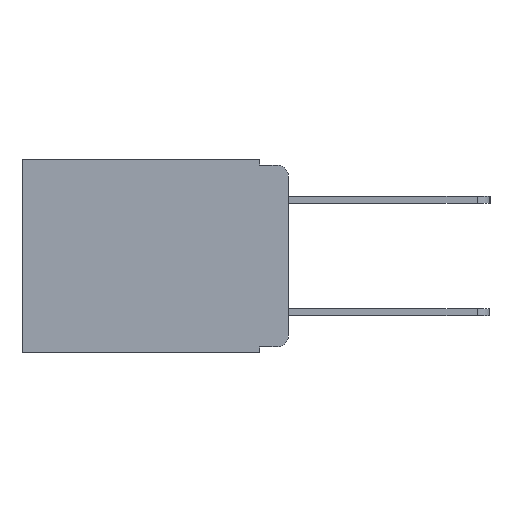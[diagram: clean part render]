
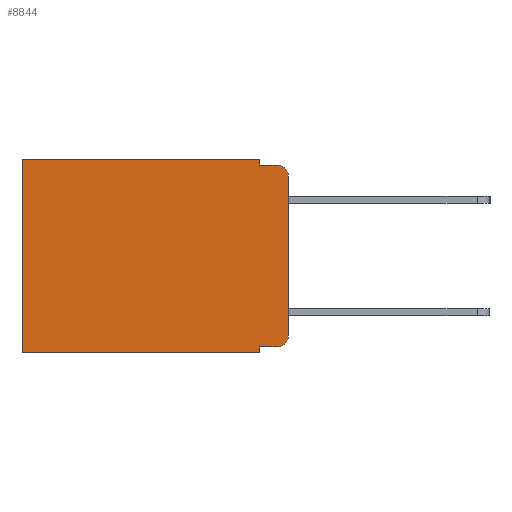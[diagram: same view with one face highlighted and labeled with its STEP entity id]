
A CAD part, left-side view. The second image highlights one B-rep face of the part: STEP entity #8844.
In plain terms, the highlighted planar face has unit normal (-1, 0, 0).
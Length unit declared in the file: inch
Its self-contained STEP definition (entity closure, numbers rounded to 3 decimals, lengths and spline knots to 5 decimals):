
#23 = FACE_OUTER_BOUND ( 'NONE', #2039, .T. ) ;
#120 = CARTESIAN_POINT ( 'NONE',  ( 0.298, 0.051, -0.333 ) ) ;
#364 = DIRECTION ( 'NONE',  ( 0., -1., 0. ) ) ;
#382 = EDGE_CURVE ( 'NONE', #1168, #11165, #4127, .T. ) ;
#595 = LINE ( 'NONE', #13211, #10138 ) ;
#816 = DIRECTION ( 'NONE',  ( 0., 0., -1. ) ) ;
#853 = DIRECTION ( 'NONE',  ( -1., 0., 0. ) ) ;
#1045 = DIRECTION ( 'NONE',  ( 0., 0., -1. ) ) ;
#1168 = VERTEX_POINT ( 'NONE', #8600 ) ;
#1632 = DIRECTION ( 'NONE',  ( 0., 1., 0. ) ) ;
#1822 = EDGE_CURVE ( 'NONE', #5927, #11089, #12730, .T. ) ;
#2039 = EDGE_LOOP ( 'NONE', ( #3342, #4807, #10661, #10383, #11116, #9831, #6508, #9892, #9722, #5983 ) ) ;
#2192 = CIRCLE ( 'NONE', #5929, 0.02 ) ;
#2300 = CARTESIAN_POINT ( 'NONE',  ( 0.298, 0.02, -0.03 ) ) ;
#2353 = VERTEX_POINT ( 'NONE', #12437 ) ;
#2358 = CARTESIAN_POINT ( 'NONE',  ( 0.298, 0.051, -0.01 ) ) ;
#2386 = CARTESIAN_POINT ( 'NONE',  ( 0.298, 0.473, 0. ) ) ;
#2470 = VECTOR ( 'NONE', #8988, 39.37008 ) ;
#2638 = LINE ( 'NONE', #6928, #6147 ) ;
#2718 = DIRECTION ( 'NONE',  ( 0., 0., -1. ) ) ;
#2736 = CARTESIAN_POINT ( 'NONE',  ( 0.298, 0., 0. ) ) ;
#2819 = EDGE_CURVE ( 'NONE', #6483, #2353, #595, .T. ) ;
#2827 = EDGE_CURVE ( 'NONE', #6483, #5071, #15735, .T. ) ;
#2848 = EDGE_CURVE ( 'NONE', #2984, #5071, #6555, .T. ) ;
#2853 = EDGE_CURVE ( 'NONE', #1168, #2984, #9769, .T. ) ;
#2872 = EDGE_CURVE ( 'NONE', #11165, #11089, #12503, .T. ) ;
#2875 = EDGE_CURVE ( 'NONE', #4786, #5927, #2638, .T. ) ;
#2893 = EDGE_CURVE ( 'NONE', #4786, #8347, #3067, .T. ) ;
#2898 = EDGE_CURVE ( 'NONE', #8347, #2353, #2192, .T. ) ;
#2984 = VERTEX_POINT ( 'NONE', #2358 ) ;
#3067 = LINE ( 'NONE', #14488, #14718 ) ;
#3342 = ORIENTED_EDGE ( 'NONE', *, *, #2819, .F. ) ;
#4068 = DIRECTION ( 'NONE',  ( 0., 0., -1. ) ) ;
#4127 = LINE ( 'NONE', #15677, #2470 ) ;
#4152 = AXIS2_PLACEMENT_3D ( 'NONE', #2300, #853, #816 ) ;
#4436 = CARTESIAN_POINT ( 'NONE',  ( 0.298, 0.02, -0.313 ) ) ;
#4786 = VERTEX_POINT ( 'NONE', #120 ) ;
#4807 = ORIENTED_EDGE ( 'NONE', *, *, #2827, .T. ) ;
#5071 = VERTEX_POINT ( 'NONE', #7488 ) ;
#5724 = CARTESIAN_POINT ( 'NONE',  ( 0.298, 0., -0.03 ) ) ;
#5927 = VERTEX_POINT ( 'NONE', #10716 ) ;
#5929 = AXIS2_PLACEMENT_3D ( 'NONE', #4436, #6004, #14410 ) ;
#5983 = ORIENTED_EDGE ( 'NONE', *, *, #2898, .T. ) ;
#5984 = VECTOR ( 'NONE', #1632, 39.37008 ) ;
#6004 = DIRECTION ( 'NONE',  ( -1., 0., 0. ) ) ;
#6147 = VECTOR ( 'NONE', #1045, 39.37008 ) ;
#6483 = VERTEX_POINT ( 'NONE', #5724 ) ;
#6508 = ORIENTED_EDGE ( 'NONE', *, *, #1822, .F. ) ;
#6555 = LINE ( 'NONE', #15197, #15394 ) ;
#6928 = CARTESIAN_POINT ( 'NONE',  ( 0.298, 0.051, 0. ) ) ;
#7488 = CARTESIAN_POINT ( 'NONE',  ( 0.298, 0.02, -0.01 ) ) ;
#7489 = CARTESIAN_POINT ( 'NONE',  ( 0.298, 0.051, 0. ) ) ;
#8347 = VERTEX_POINT ( 'NONE', #14146 ) ;
#8600 = CARTESIAN_POINT ( 'NONE',  ( 0.298, 0.051, 0. ) ) ;
#8844 = ADVANCED_FACE ( 'NONE', ( #23 ), #15834, .F. ) ;
#8868 = CARTESIAN_POINT ( 'NONE',  ( 0.298, 0.473, 0. ) ) ;
#8988 = DIRECTION ( 'NONE',  ( 0., 1., 0. ) ) ;
#9368 = VECTOR ( 'NONE', #2718, 39.37008 ) ;
#9722 = ORIENTED_EDGE ( 'NONE', *, *, #2893, .T. ) ;
#9769 = LINE ( 'NONE', #7489, #9368 ) ;
#9804 = DIRECTION ( 'NONE',  ( 0., -1., 0. ) ) ;
#9831 = ORIENTED_EDGE ( 'NONE', *, *, #2872, .T. ) ;
#9892 = ORIENTED_EDGE ( 'NONE', *, *, #2875, .F. ) ;
#10138 = VECTOR ( 'NONE', #13155, 39.37008 ) ;
#10383 = ORIENTED_EDGE ( 'NONE', *, *, #2853, .F. ) ;
#10661 = ORIENTED_EDGE ( 'NONE', *, *, #2848, .F. ) ;
#10707 = CARTESIAN_POINT ( 'NONE',  ( 0.298, 0., -0.343 ) ) ;
#10716 = CARTESIAN_POINT ( 'NONE',  ( 0.298, 0.051, -0.343 ) ) ;
#10938 = AXIS2_PLACEMENT_3D ( 'NONE', #2736, #11440, #4068 ) ;
#11089 = VERTEX_POINT ( 'NONE', #13414 ) ;
#11116 = ORIENTED_EDGE ( 'NONE', *, *, #382, .T. ) ;
#11165 = VERTEX_POINT ( 'NONE', #8868 ) ;
#11440 = DIRECTION ( 'NONE',  ( 1., 0., 0. ) ) ;
#12232 = DIRECTION ( 'NONE',  ( 0., 0., -1. ) ) ;
#12437 = CARTESIAN_POINT ( 'NONE',  ( 0.298, 0., -0.313 ) ) ;
#12503 = LINE ( 'NONE', #2386, #15050 ) ;
#12730 = LINE ( 'NONE', #10707, #5984 ) ;
#13155 = DIRECTION ( 'NONE',  ( 0., 0., -1. ) ) ;
#13211 = CARTESIAN_POINT ( 'NONE',  ( 0.298, 0., 0. ) ) ;
#13414 = CARTESIAN_POINT ( 'NONE',  ( 0.298, 0.473, -0.343 ) ) ;
#14146 = CARTESIAN_POINT ( 'NONE',  ( 0.298, 0.02, -0.333 ) ) ;
#14410 = DIRECTION ( 'NONE',  ( 0., 0., -1. ) ) ;
#14488 = CARTESIAN_POINT ( 'NONE',  ( 0.298, 0.051, -0.333 ) ) ;
#14718 = VECTOR ( 'NONE', #9804, 39.37008 ) ;
#15050 = VECTOR ( 'NONE', #12232, 39.37008 ) ;
#15197 = CARTESIAN_POINT ( 'NONE',  ( 0.298, 0.051, -0.01 ) ) ;
#15394 = VECTOR ( 'NONE', #364, 39.37008 ) ;
#15677 = CARTESIAN_POINT ( 'NONE',  ( 0.298, 0., 0. ) ) ;
#15735 = CIRCLE ( 'NONE', #4152, 0.02 ) ;
#15834 = PLANE ( 'NONE',  #10938 ) ;
